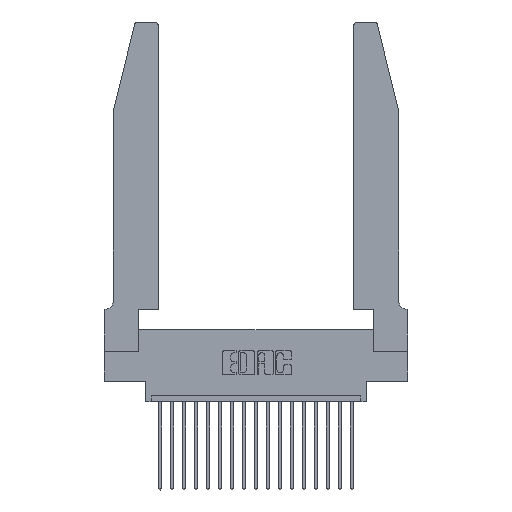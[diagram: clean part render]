
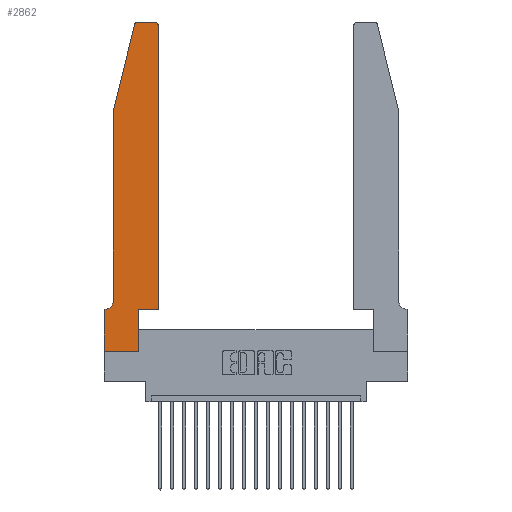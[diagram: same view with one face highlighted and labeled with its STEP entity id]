
A CAD part, top view. The second image highlights one B-rep face of the part: STEP entity #2862.
In plain terms, the highlighted planar face has unit normal (0, 0, 1).
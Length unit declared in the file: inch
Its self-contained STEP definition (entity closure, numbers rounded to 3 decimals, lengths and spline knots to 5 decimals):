
#43 = CARTESIAN_POINT ( 'NONE',  ( 0.0755, 0.35, 0.37 ) ) ;
#240 = EDGE_CURVE ( 'NONE', #4803, #6778, #18486, .T. ) ;
#784 = DIRECTION ( 'NONE',  ( 0., -1., 0. ) ) ;
#882 = EDGE_CURVE ( 'NONE', #19796, #9815, #9770, .T. ) ;
#921 = CARTESIAN_POINT ( 'NONE',  ( 0.2865, 0.35, 0.37 ) ) ;
#1366 = DIRECTION ( 'NONE',  ( 1., 0., 0. ) ) ;
#1694 = VECTOR ( 'NONE', #12468, 39.37008 ) ;
#2054 = ORIENTED_EDGE ( 'NONE', *, *, #882, .T. ) ;
#2105 = CARTESIAN_POINT ( 'NONE',  ( 0.0755, 0.42, 0.37 ) ) ;
#2223 = CARTESIAN_POINT ( 'NONE',  ( 0.0755, 2., 0.37 ) ) ;
#2260 = AXIS2_PLACEMENT_3D ( 'NONE', #10323, #18448, #18313 ) ;
#2580 = VERTEX_POINT ( 'NONE', #19502 ) ;
#2619 = LINE ( 'NONE', #8379, #10479 ) ;
#2623 = CARTESIAN_POINT ( 'NONE',  ( 0.4505, 2.72, 0.37 ) ) ;
#2624 = ORIENTED_EDGE ( 'NONE', *, *, #8992, .T. ) ;
#2862 = ADVANCED_FACE ( 'NONE', ( #15624 ), #19065, .T. ) ;
#2976 = VECTOR ( 'NONE', #6305, 39.37008 ) ;
#3160 = VERTEX_POINT ( 'NONE', #15862 ) ;
#3300 = EDGE_CURVE ( 'NONE', #20059, #13039, #17671, .T. ) ;
#3348 = CARTESIAN_POINT ( 'NONE',  ( 0.25487, 2.72718, 0.37 ) ) ;
#3504 = LINE ( 'NONE', #4691, #2976 ) ;
#3710 = ORIENTED_EDGE ( 'NONE', *, *, #16825, .T. ) ;
#3915 = VECTOR ( 'NONE', #784, 39.37008 ) ;
#4122 = LINE ( 'NONE', #9278, #13221 ) ;
#4171 = CARTESIAN_POINT ( 'NONE',  ( 0.0755, 2., 0.37 ) ) ;
#4186 = ORIENTED_EDGE ( 'NONE', *, *, #19588, .T. ) ;
#4357 = DIRECTION ( 'NONE',  ( -0.239, -0.971, 0. ) ) ;
#4443 = CARTESIAN_POINT ( 'NONE',  ( 0., 0., 0.37 ) ) ;
#4530 = CARTESIAN_POINT ( 'NONE',  ( 0., 0.35, 0.37 ) ) ;
#4691 = CARTESIAN_POINT ( 'NONE',  ( 0.2605, 2.75, 0.37 ) ) ;
#4803 = VERTEX_POINT ( 'NONE', #14558 ) ;
#5185 = CARTESIAN_POINT ( 'NONE',  ( 0., 0., 0.37 ) ) ;
#5690 = DIRECTION ( 'NONE',  ( 1., 0., 0. ) ) ;
#5871 = CARTESIAN_POINT ( 'NONE',  ( 0.2865, 0., 0.37 ) ) ;
#6083 = CIRCLE ( 'NONE', #12484, 0.03 ) ;
#6234 = DIRECTION ( 'NONE',  ( -1., 0., 0. ) ) ;
#6291 = ORIENTED_EDGE ( 'NONE', *, *, #14192, .T. ) ;
#6305 = DIRECTION ( 'NONE',  ( -1., 0., 0. ) ) ;
#6778 = VERTEX_POINT ( 'NONE', #3348 ) ;
#6781 = VERTEX_POINT ( 'NONE', #11189 ) ;
#7025 = LINE ( 'NONE', #5185, #15095 ) ;
#7050 = EDGE_LOOP ( 'NONE', ( #4186, #13234, #19051, #16949, #2054, #6291, #7270, #2624, #19879, #3710, #12664, #9554 ) ) ;
#7262 = CARTESIAN_POINT ( 'NONE',  ( 0.0055, 0.35, 0.37 ) ) ;
#7270 = ORIENTED_EDGE ( 'NONE', *, *, #14997, .T. ) ;
#7699 = VERTEX_POINT ( 'NONE', #2623 ) ;
#7766 = CARTESIAN_POINT ( 'NONE',  ( 0.0055, 0.42, 0.37 ) ) ;
#8222 = EDGE_CURVE ( 'NONE', #7699, #3160, #6083, .T. ) ;
#8379 = CARTESIAN_POINT ( 'NONE',  ( 0.4505, 0.35, 0.37 ) ) ;
#8968 = LINE ( 'NONE', #4171, #3915 ) ;
#8992 = EDGE_CURVE ( 'NONE', #15668, #20059, #11868, .T. ) ;
#9206 = CARTESIAN_POINT ( 'NONE',  ( 0., 0., 0.37 ) ) ;
#9278 = CARTESIAN_POINT ( 'NONE',  ( 0.0755, 2., 0.37 ) ) ;
#9554 = ORIENTED_EDGE ( 'NONE', *, *, #8222, .T. ) ;
#9770 = CIRCLE ( 'NONE', #18254, 0.07 ) ;
#9815 = VERTEX_POINT ( 'NONE', #7262 ) ;
#9994 = DIRECTION ( 'NONE',  ( 1., 0., 0. ) ) ;
#10313 = EDGE_CURVE ( 'NONE', #2580, #7699, #12824, .T. ) ;
#10323 = CARTESIAN_POINT ( 'NONE',  ( 0.284, 2.72, 0.37 ) ) ;
#10479 = VECTOR ( 'NONE', #9994, 39.37008 ) ;
#10756 = VERTEX_POINT ( 'NONE', #2223 ) ;
#11189 = CARTESIAN_POINT ( 'NONE',  ( 0., 0.35, 0.37 ) ) ;
#11304 = CARTESIAN_POINT ( 'NONE',  ( 0.2865, 0.35, 0.37 ) ) ;
#11343 = DIRECTION ( 'NONE',  ( -1., 0., 0. ) ) ;
#11868 = LINE ( 'NONE', #9206, #1694 ) ;
#11897 = EDGE_CURVE ( 'NONE', #10756, #19796, #8968, .T. ) ;
#11989 = CARTESIAN_POINT ( 'NONE',  ( 0.4205, 2.72, 0.37 ) ) ;
#12468 = DIRECTION ( 'NONE',  ( 1., 0., 0. ) ) ;
#12484 = AXIS2_PLACEMENT_3D ( 'NONE', #11989, #18755, #5690 ) ;
#12535 = AXIS2_PLACEMENT_3D ( 'NONE', #4530, #14262, #1366 ) ;
#12664 = ORIENTED_EDGE ( 'NONE', *, *, #10313, .T. ) ;
#12824 = LINE ( 'NONE', #15374, #20944 ) ;
#13039 = VERTEX_POINT ( 'NONE', #921 ) ;
#13185 = EDGE_CURVE ( 'NONE', #6778, #10756, #4122, .T. ) ;
#13221 = VECTOR ( 'NONE', #4357, 39.37008 ) ;
#13234 = ORIENTED_EDGE ( 'NONE', *, *, #240, .T. ) ;
#13326 = VECTOR ( 'NONE', #20843, 39.37008 ) ;
#14192 = EDGE_CURVE ( 'NONE', #9815, #6781, #15953, .T. ) ;
#14262 = DIRECTION ( 'NONE',  ( 0., 0., 1. ) ) ;
#14558 = CARTESIAN_POINT ( 'NONE',  ( 0.284, 2.75, 0.37 ) ) ;
#14592 = DIRECTION ( 'NONE',  ( 0., -1., 0. ) ) ;
#14997 = EDGE_CURVE ( 'NONE', #6781, #15668, #7025, .T. ) ;
#15095 = VECTOR ( 'NONE', #14592, 39.37008 ) ;
#15374 = CARTESIAN_POINT ( 'NONE',  ( 0.4505, 0.35, 0.37 ) ) ;
#15624 = FACE_OUTER_BOUND ( 'NONE', #7050, .T. ) ;
#15668 = VERTEX_POINT ( 'NONE', #4443 ) ;
#15862 = CARTESIAN_POINT ( 'NONE',  ( 0.4205, 2.75, 0.37 ) ) ;
#15890 = DIRECTION ( 'NONE',  ( 0., 0., -1. ) ) ;
#15953 = LINE ( 'NONE', #43, #17756 ) ;
#16825 = EDGE_CURVE ( 'NONE', #13039, #2580, #2619, .T. ) ;
#16919 = DIRECTION ( 'NONE',  ( 0., 1., 0. ) ) ;
#16949 = ORIENTED_EDGE ( 'NONE', *, *, #11897, .T. ) ;
#17671 = LINE ( 'NONE', #11304, #13326 ) ;
#17756 = VECTOR ( 'NONE', #11343, 39.37008 ) ;
#18254 = AXIS2_PLACEMENT_3D ( 'NONE', #7766, #15890, #6234 ) ;
#18313 = DIRECTION ( 'NONE',  ( 1., 0., 0. ) ) ;
#18448 = DIRECTION ( 'NONE',  ( 0., 0., 1. ) ) ;
#18486 = CIRCLE ( 'NONE', #2260, 0.03 ) ;
#18755 = DIRECTION ( 'NONE',  ( 0., 0., 1. ) ) ;
#19051 = ORIENTED_EDGE ( 'NONE', *, *, #13185, .T. ) ;
#19065 = PLANE ( 'NONE',  #12535 ) ;
#19502 = CARTESIAN_POINT ( 'NONE',  ( 0.4505, 0.35, 0.37 ) ) ;
#19588 = EDGE_CURVE ( 'NONE', #3160, #4803, #3504, .T. ) ;
#19796 = VERTEX_POINT ( 'NONE', #2105 ) ;
#19879 = ORIENTED_EDGE ( 'NONE', *, *, #3300, .T. ) ;
#20059 = VERTEX_POINT ( 'NONE', #5871 ) ;
#20843 = DIRECTION ( 'NONE',  ( 0., 1., 0. ) ) ;
#20944 = VECTOR ( 'NONE', #16919, 39.37008 ) ;
